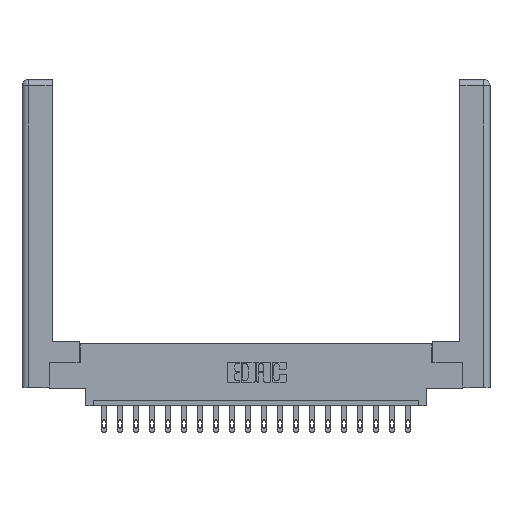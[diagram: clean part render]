
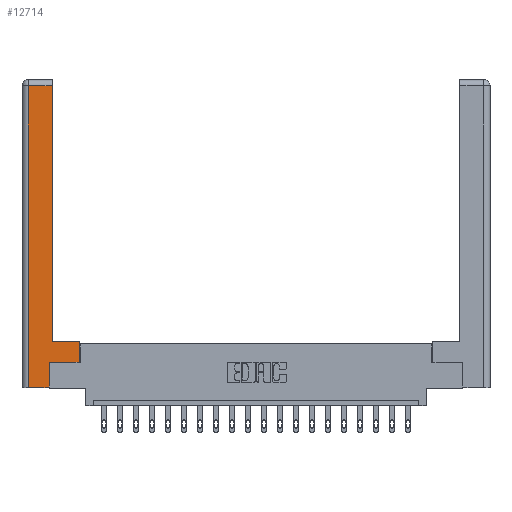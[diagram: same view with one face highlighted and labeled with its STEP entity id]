
A CAD part, top view. The second image highlights one B-rep face of the part: STEP entity #12714.
In plain terms, the highlighted planar face has unit normal (0, 0, 1).
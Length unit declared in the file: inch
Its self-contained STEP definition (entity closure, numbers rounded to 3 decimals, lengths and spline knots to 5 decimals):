
#105 = DIRECTION ( 'NONE',  ( 1., 0., 0. ) ) ;
#238 = EDGE_LOOP ( 'NONE', ( #13635, #16573, #15814, #6103, #7827, #9274, #19784, #11929 ) ) ;
#251 = VERTEX_POINT ( 'NONE', #13924 ) ;
#338 = DIRECTION ( 'NONE',  ( -1., 0., 0. ) ) ;
#1483 = EDGE_CURVE ( 'NONE', #13782, #4068, #11579, .T. ) ;
#2759 = VERTEX_POINT ( 'NONE', #15691 ) ;
#3405 = VECTOR ( 'NONE', #14557, 39.37008 ) ;
#3430 = VECTOR ( 'NONE', #15075, 39.37008 ) ;
#3492 = CARTESIAN_POINT ( 'NONE',  ( 0.565, 0.45, 0. ) ) ;
#3907 = CARTESIAN_POINT ( 'NONE',  ( 0.0615, 0., 0. ) ) ;
#4009 = CARTESIAN_POINT ( 'NONE',  ( 0.295, 0.45, 0. ) ) ;
#4068 = VERTEX_POINT ( 'NONE', #6966 ) ;
#4159 = LINE ( 'NONE', #17780, #3405 ) ;
#4173 = DIRECTION ( 'NONE',  ( 0., 0., -1. ) ) ;
#4303 = PLANE ( 'NONE',  #5671 ) ;
#5671 = AXIS2_PLACEMENT_3D ( 'NONE', #18255, #4173, #8798 ) ;
#6103 = ORIENTED_EDGE ( 'NONE', *, *, #19477, .T. ) ;
#6124 = CARTESIAN_POINT ( 'NONE',  ( 0.295, 2.94, 0. ) ) ;
#6899 = CARTESIAN_POINT ( 'NONE',  ( 0.565, 0.45, 0. ) ) ;
#6927 = CARTESIAN_POINT ( 'NONE',  ( 0.265, 0., 0. ) ) ;
#6966 = CARTESIAN_POINT ( 'NONE',  ( 0.0615, 0., 0. ) ) ;
#7316 = VECTOR ( 'NONE', #17663, 39.37008 ) ;
#7335 = VECTOR ( 'NONE', #105, 39.37008 ) ;
#7478 = VECTOR ( 'NONE', #338, 39.37008 ) ;
#7827 = ORIENTED_EDGE ( 'NONE', *, *, #13522, .T. ) ;
#7852 = LINE ( 'NONE', #18512, #15288 ) ;
#8319 = LINE ( 'NONE', #15986, #7335 ) ;
#8750 = LINE ( 'NONE', #15357, #19838 ) ;
#8798 = DIRECTION ( 'NONE',  ( -1., 0., 0. ) ) ;
#9274 = ORIENTED_EDGE ( 'NONE', *, *, #19889, .T. ) ;
#10266 = CARTESIAN_POINT ( 'NONE',  ( 0.295, 3., 0. ) ) ;
#10552 = VERTEX_POINT ( 'NONE', #6899 ) ;
#11238 = LINE ( 'NONE', #3492, #7316 ) ;
#11579 = LINE ( 'NONE', #3907, #18991 ) ;
#11673 = LINE ( 'NONE', #17651, #7478 ) ;
#11929 = ORIENTED_EDGE ( 'NONE', *, *, #12555, .T. ) ;
#12015 = DIRECTION ( 'NONE',  ( 0., 1., 0. ) ) ;
#12161 = DIRECTION ( 'NONE',  ( 1., 0., 0. ) ) ;
#12555 = EDGE_CURVE ( 'NONE', #10552, #16263, #4159, .T. ) ;
#12622 = VERTEX_POINT ( 'NONE', #6927 ) ;
#12714 = ADVANCED_FACE ( 'NONE', ( #13293 ), #4303, .F. ) ;
#13253 = CARTESIAN_POINT ( 'NONE',  ( 0.0615, 2.94, 0. ) ) ;
#13293 = FACE_OUTER_BOUND ( 'NONE', #238, .T. ) ;
#13522 = EDGE_CURVE ( 'NONE', #12622, #2759, #8750, .T. ) ;
#13635 = ORIENTED_EDGE ( 'NONE', *, *, #17099, .T. ) ;
#13782 = VERTEX_POINT ( 'NONE', #13253 ) ;
#13924 = CARTESIAN_POINT ( 'NONE',  ( 0.565, 0.245, 0. ) ) ;
#14333 = EDGE_CURVE ( 'NONE', #15302, #13782, #11673, .T. ) ;
#14557 = DIRECTION ( 'NONE',  ( -1., 0., 0. ) ) ;
#14843 = DIRECTION ( 'NONE',  ( 0., -1., 0. ) ) ;
#15075 = DIRECTION ( 'NONE',  ( 0., 1., 0. ) ) ;
#15288 = VECTOR ( 'NONE', #12161, 39.37008 ) ;
#15302 = VERTEX_POINT ( 'NONE', #6124 ) ;
#15357 = CARTESIAN_POINT ( 'NONE',  ( 0.265, 0.245, 0. ) ) ;
#15691 = CARTESIAN_POINT ( 'NONE',  ( 0.265, 0.245, 0. ) ) ;
#15814 = ORIENTED_EDGE ( 'NONE', *, *, #1483, .T. ) ;
#15986 = CARTESIAN_POINT ( 'NONE',  ( 0.565, 0.245, 0. ) ) ;
#16263 = VERTEX_POINT ( 'NONE', #4009 ) ;
#16573 = ORIENTED_EDGE ( 'NONE', *, *, #14333, .T. ) ;
#17099 = EDGE_CURVE ( 'NONE', #16263, #15302, #18732, .T. ) ;
#17651 = CARTESIAN_POINT ( 'NONE',  ( 0.0615, 2.94, 0. ) ) ;
#17663 = DIRECTION ( 'NONE',  ( 0., 1., 0. ) ) ;
#17780 = CARTESIAN_POINT ( 'NONE',  ( 0.295, 0.45, 0. ) ) ;
#18255 = CARTESIAN_POINT ( 'NONE',  ( 0., 0., 0. ) ) ;
#18512 = CARTESIAN_POINT ( 'NONE',  ( 0.265, 0., 0. ) ) ;
#18575 = EDGE_CURVE ( 'NONE', #251, #10552, #11238, .T. ) ;
#18732 = LINE ( 'NONE', #10266, #3430 ) ;
#18991 = VECTOR ( 'NONE', #14843, 39.37008 ) ;
#19477 = EDGE_CURVE ( 'NONE', #4068, #12622, #7852, .T. ) ;
#19784 = ORIENTED_EDGE ( 'NONE', *, *, #18575, .T. ) ;
#19838 = VECTOR ( 'NONE', #12015, 39.37008 ) ;
#19889 = EDGE_CURVE ( 'NONE', #2759, #251, #8319, .T. ) ;
